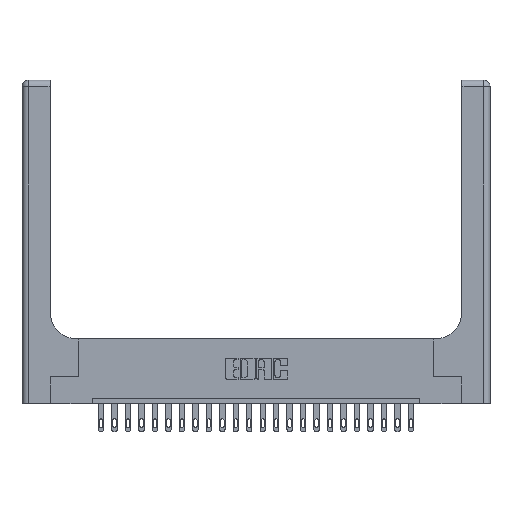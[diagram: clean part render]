
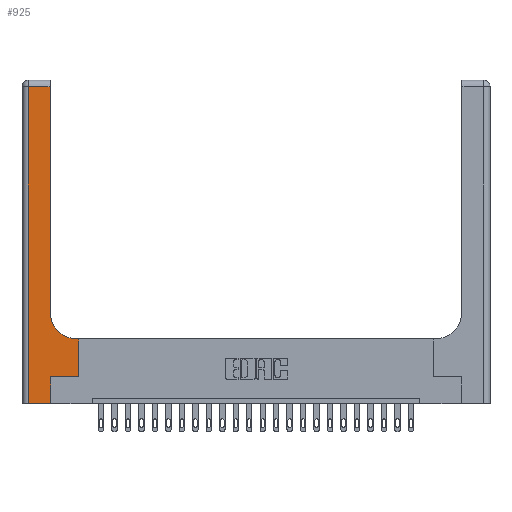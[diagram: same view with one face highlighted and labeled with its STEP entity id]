
A CAD part, top view. The second image highlights one B-rep face of the part: STEP entity #925.
In plain terms, the highlighted planar face has unit normal (0, 0, 1).
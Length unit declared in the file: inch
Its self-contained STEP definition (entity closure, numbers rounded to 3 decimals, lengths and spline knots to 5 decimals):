
#25 = CARTESIAN_POINT ( 'NONE',  ( 0.06, 0., 0.37 ) ) ;
#135 = CARTESIAN_POINT ( 'NONE',  ( 0.26, 2.94, 0.37 ) ) ;
#180 = LINE ( 'NONE', #6867, #18952 ) ;
#344 = CARTESIAN_POINT ( 'NONE',  ( 0., 2.94, 0.37 ) ) ;
#793 = EDGE_LOOP ( 'NONE', ( #21153, #11330, #12621, #18596, #8492, #21875, #3678, #19556, #7232 ) ) ;
#828 = DIRECTION ( 'NONE',  ( -1., 0., 0. ) ) ;
#847 = CARTESIAN_POINT ( 'NONE',  ( 0.51, 0.85, 0.37 ) ) ;
#925 = ADVANCED_FACE ( 'NONE', ( #15038 ), #4513, .F. ) ;
#2084 = DIRECTION ( 'NONE',  ( -1., 0., 0. ) ) ;
#2091 = EDGE_CURVE ( 'NONE', #17040, #12700, #16161, .T. ) ;
#2356 = EDGE_CURVE ( 'NONE', #12700, #5916, #15680, .T. ) ;
#2371 = CARTESIAN_POINT ( 'NONE',  ( 0.528, 0.25, 0.37 ) ) ;
#2442 = VERTEX_POINT ( 'NONE', #2371 ) ;
#3093 = DIRECTION ( 'NONE',  ( 1., 0., 0. ) ) ;
#3678 = ORIENTED_EDGE ( 'NONE', *, *, #19574, .T. ) ;
#3978 = VECTOR ( 'NONE', #7387, 39.37008 ) ;
#4274 = EDGE_CURVE ( 'NONE', #11101, #17580, #20956, .T. ) ;
#4513 = PLANE ( 'NONE',  #13850 ) ;
#5379 = CARTESIAN_POINT ( 'NONE',  ( 0.06, 3., 0.37 ) ) ;
#5552 = LINE ( 'NONE', #21425, #22637 ) ;
#5568 = DIRECTION ( 'NONE',  ( 1., 0., 0. ) ) ;
#5904 = CARTESIAN_POINT ( 'NONE',  ( 0.265, 0.25, 0.37 ) ) ;
#5916 = VERTEX_POINT ( 'NONE', #25 ) ;
#6090 = EDGE_CURVE ( 'NONE', #17580, #17040, #19665, .T. ) ;
#6125 = VECTOR ( 'NONE', #5568, 39.37008 ) ;
#6842 = CARTESIAN_POINT ( 'NONE',  ( 0.51, 0.6, 0.37 ) ) ;
#6867 = CARTESIAN_POINT ( 'NONE',  ( 0.528, 0.25, 0.37 ) ) ;
#7232 = ORIENTED_EDGE ( 'NONE', *, *, #4274, .T. ) ;
#7387 = DIRECTION ( 'NONE',  ( -1., 0., 0. ) ) ;
#7907 = DIRECTION ( 'NONE',  ( 0., 0., -1. ) ) ;
#8195 = CARTESIAN_POINT ( 'NONE',  ( 0.06, 2.94, 0.37 ) ) ;
#8473 = DIRECTION ( 'NONE',  ( 1., 0., 0. ) ) ;
#8492 = ORIENTED_EDGE ( 'NONE', *, *, #9518, .T. ) ;
#8839 = DIRECTION ( 'NONE',  ( 0., 1., 0. ) ) ;
#9422 = CARTESIAN_POINT ( 'NONE',  ( 0.265, 0.25, 0.37 ) ) ;
#9518 = EDGE_CURVE ( 'NONE', #20795, #11927, #14921, .T. ) ;
#9594 = VECTOR ( 'NONE', #19374, 39.37008 ) ;
#9610 = CARTESIAN_POINT ( 'NONE',  ( 0.265, 0., 0.37 ) ) ;
#10783 = LINE ( 'NONE', #5904, #6125 ) ;
#11101 = VERTEX_POINT ( 'NONE', #6842 ) ;
#11330 = ORIENTED_EDGE ( 'NONE', *, *, #2091, .T. ) ;
#11927 = VERTEX_POINT ( 'NONE', #9422 ) ;
#12621 = ORIENTED_EDGE ( 'NONE', *, *, #2356, .T. ) ;
#12677 = EDGE_CURVE ( 'NONE', #5916, #20795, #13617, .T. ) ;
#12700 = VERTEX_POINT ( 'NONE', #8195 ) ;
#12971 = CARTESIAN_POINT ( 'NONE',  ( 0.26, 3., 0.37 ) ) ;
#13469 = CARTESIAN_POINT ( 'NONE',  ( 0.265, 0., 0.37 ) ) ;
#13531 = DIRECTION ( 'NONE',  ( 0., 1., 0. ) ) ;
#13617 = LINE ( 'NONE', #17299, #21597 ) ;
#13850 = AXIS2_PLACEMENT_3D ( 'NONE', #20490, #16658, #828 ) ;
#14376 = VECTOR ( 'NONE', #17923, 39.37008 ) ;
#14921 = LINE ( 'NONE', #9610, #16306 ) ;
#15038 = FACE_OUTER_BOUND ( 'NONE', #793, .T. ) ;
#15680 = LINE ( 'NONE', #5379, #9594 ) ;
#16161 = LINE ( 'NONE', #344, #3978 ) ;
#16306 = VECTOR ( 'NONE', #13531, 39.37008 ) ;
#16658 = DIRECTION ( 'NONE',  ( 0., 0., -1. ) ) ;
#17021 = EDGE_CURVE ( 'NONE', #18851, #11101, #5552, .T. ) ;
#17040 = VERTEX_POINT ( 'NONE', #135 ) ;
#17299 = CARTESIAN_POINT ( 'NONE',  ( 0., 0., 0.37 ) ) ;
#17580 = VERTEX_POINT ( 'NONE', #21965 ) ;
#17923 = DIRECTION ( 'NONE',  ( 0., 1., 0. ) ) ;
#18596 = ORIENTED_EDGE ( 'NONE', *, *, #12677, .T. ) ;
#18851 = VERTEX_POINT ( 'NONE', #22078 ) ;
#18952 = VECTOR ( 'NONE', #8839, 39.37008 ) ;
#19374 = DIRECTION ( 'NONE',  ( 0., -1., 0. ) ) ;
#19556 = ORIENTED_EDGE ( 'NONE', *, *, #17021, .T. ) ;
#19574 = EDGE_CURVE ( 'NONE', #2442, #18851, #180, .T. ) ;
#19665 = LINE ( 'NONE', #12971, #14376 ) ;
#20490 = CARTESIAN_POINT ( 'NONE',  ( 0., 3., 0.37 ) ) ;
#20795 = VERTEX_POINT ( 'NONE', #13469 ) ;
#20956 = CIRCLE ( 'NONE', #21331, 0.25 ) ;
#21153 = ORIENTED_EDGE ( 'NONE', *, *, #6090, .T. ) ;
#21331 = AXIS2_PLACEMENT_3D ( 'NONE', #847, #7907, #8473 ) ;
#21425 = CARTESIAN_POINT ( 'NONE',  ( 0.26, 0.6, 0.37 ) ) ;
#21597 = VECTOR ( 'NONE', #3093, 39.37008 ) ;
#21875 = ORIENTED_EDGE ( 'NONE', *, *, #22639, .T. ) ;
#21965 = CARTESIAN_POINT ( 'NONE',  ( 0.26, 0.85, 0.37 ) ) ;
#22078 = CARTESIAN_POINT ( 'NONE',  ( 0.528, 0.6, 0.37 ) ) ;
#22637 = VECTOR ( 'NONE', #2084, 39.37008 ) ;
#22639 = EDGE_CURVE ( 'NONE', #11927, #2442, #10783, .T. ) ;
